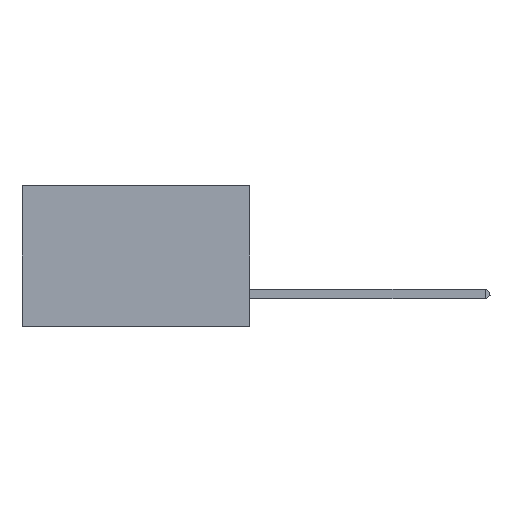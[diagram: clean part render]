
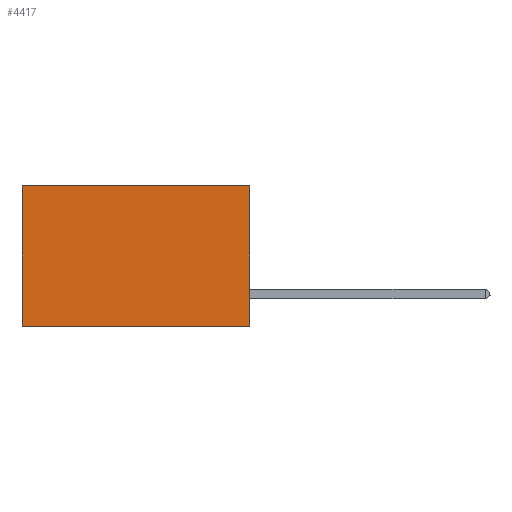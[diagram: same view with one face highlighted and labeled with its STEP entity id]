
A CAD part, left-side view. The second image highlights one B-rep face of the part: STEP entity #4417.
In plain terms, the highlighted planar face has unit normal (-1, 0, 0).
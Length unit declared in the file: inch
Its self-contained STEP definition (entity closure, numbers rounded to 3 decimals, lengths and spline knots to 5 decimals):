
#620 = CARTESIAN_POINT ( 'NONE',  ( 0.2875, 0.6, 0. ) ) ;
#869 = CARTESIAN_POINT ( 'NONE',  ( 0.2875, 0., -0.37 ) ) ;
#1440 = VECTOR ( 'NONE', #5839, 39.37008 ) ;
#1753 = LINE ( 'NONE', #8809, #15020 ) ;
#1812 = ORIENTED_EDGE ( 'NONE', *, *, #11570, .F. ) ;
#2109 = EDGE_LOOP ( 'NONE', ( #15876, #7566, #1812, #4152 ) ) ;
#2232 = DIRECTION ( 'NONE',  ( 0., 0., -1. ) ) ;
#3622 = CARTESIAN_POINT ( 'NONE',  ( 0.2875, 0., 0. ) ) ;
#3906 = VERTEX_POINT ( 'NONE', #869 ) ;
#4152 = ORIENTED_EDGE ( 'NONE', *, *, #11409, .T. ) ;
#4417 = ADVANCED_FACE ( 'NONE', ( #13278 ), #5836, .F. ) ;
#4483 = CARTESIAN_POINT ( 'NONE',  ( 0.2875, 0., 0. ) ) ;
#5025 = DIRECTION ( 'NONE',  ( 0., 0., -1. ) ) ;
#5093 = EDGE_CURVE ( 'NONE', #7556, #7229, #1753, .T. ) ;
#5424 = DIRECTION ( 'NONE',  ( 0., 0., -1. ) ) ;
#5589 = LINE ( 'NONE', #3622, #9269 ) ;
#5836 = PLANE ( 'NONE',  #8445 ) ;
#5839 = DIRECTION ( 'NONE',  ( 0., 1., 0. ) ) ;
#7229 = VERTEX_POINT ( 'NONE', #13855 ) ;
#7556 = VERTEX_POINT ( 'NONE', #620 ) ;
#7566 = ORIENTED_EDGE ( 'NONE', *, *, #8004, .F. ) ;
#8004 = EDGE_CURVE ( 'NONE', #3906, #7229, #8206, .T. ) ;
#8206 = LINE ( 'NONE', #13212, #1440 ) ;
#8402 = CARTESIAN_POINT ( 'NONE',  ( 0.2875, 0., 0. ) ) ;
#8445 = AXIS2_PLACEMENT_3D ( 'NONE', #8402, #8458, #2232 ) ;
#8458 = DIRECTION ( 'NONE',  ( 1., 0., 0. ) ) ;
#8809 = CARTESIAN_POINT ( 'NONE',  ( 0.2875, 0.6, 0. ) ) ;
#9269 = VECTOR ( 'NONE', #12244, 39.37008 ) ;
#10983 = VECTOR ( 'NONE', #5025, 39.37008 ) ;
#11409 = EDGE_CURVE ( 'NONE', #12377, #7556, #5589, .T. ) ;
#11570 = EDGE_CURVE ( 'NONE', #12377, #3906, #11763, .T. ) ;
#11763 = LINE ( 'NONE', #12352, #10983 ) ;
#12244 = DIRECTION ( 'NONE',  ( 0., 1., 0. ) ) ;
#12352 = CARTESIAN_POINT ( 'NONE',  ( 0.2875, 0., 0. ) ) ;
#12377 = VERTEX_POINT ( 'NONE', #4483 ) ;
#13212 = CARTESIAN_POINT ( 'NONE',  ( 0.2875, 0., -0.37 ) ) ;
#13278 = FACE_OUTER_BOUND ( 'NONE', #2109, .T. ) ;
#13855 = CARTESIAN_POINT ( 'NONE',  ( 0.2875, 0.6, -0.37 ) ) ;
#15020 = VECTOR ( 'NONE', #5424, 39.37008 ) ;
#15876 = ORIENTED_EDGE ( 'NONE', *, *, #5093, .T. ) ;
